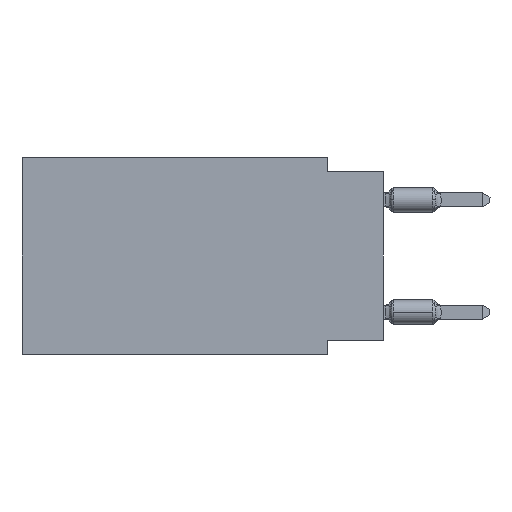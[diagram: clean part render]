
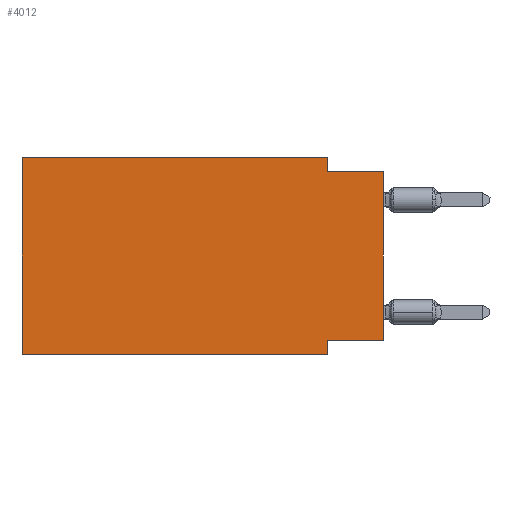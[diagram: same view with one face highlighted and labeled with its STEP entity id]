
A CAD part, left-side view. The second image highlights one B-rep face of the part: STEP entity #4012.
In plain terms, the highlighted planar face has unit normal (-1, 0, 0).
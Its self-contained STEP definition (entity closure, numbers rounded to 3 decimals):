
#630 = VERTEX_POINT ( 'NONE', #11564 ) ;
#721 = CARTESIAN_POINT ( 'NONE',  ( 0., 0., 0. ) ) ;
#818 = ORIENTED_EDGE ( 'NONE', *, *, #9635, .F. ) ;
#1525 = EDGE_CURVE ( 'NONE', #3628, #630, #20084, .T. ) ;
#1866 = EDGE_CURVE ( 'NONE', #13957, #18726, #4700, .T. ) ;
#2178 = EDGE_CURVE ( 'NONE', #13686, #16543, #19381, .T. ) ;
#2636 = VERTEX_POINT ( 'NONE', #3783 ) ;
#2865 = CARTESIAN_POINT ( 'NONE',  ( 0., 0., -8.255 ) ) ;
#2909 = DIRECTION ( 'NONE',  ( 1., 0., 0. ) ) ;
#3628 = VERTEX_POINT ( 'NONE', #11197 ) ;
#3767 = CARTESIAN_POINT ( 'NONE',  ( 0., 0., -0.635 ) ) ;
#3783 = CARTESIAN_POINT ( 'NONE',  ( 0., 2.54, 0. ) ) ;
#4012 = ADVANCED_FACE ( 'NONE', ( #11063 ), #17591, .F. ) ;
#4035 = VECTOR ( 'NONE', #10597, 1000. ) ;
#4369 = EDGE_CURVE ( 'NONE', #2636, #3628, #6198, .T. ) ;
#4674 = CARTESIAN_POINT ( 'NONE',  ( 0., 2.54, -8.89 ) ) ;
#4700 = LINE ( 'NONE', #11255, #20551 ) ;
#5410 = VECTOR ( 'NONE', #14051, 1000. ) ;
#5813 = CARTESIAN_POINT ( 'NONE',  ( 0., 16.383, 0. ) ) ;
#5863 = LINE ( 'NONE', #8883, #18308 ) ;
#5878 = ORIENTED_EDGE ( 'NONE', *, *, #2178, .F. ) ;
#6198 = LINE ( 'NONE', #20715, #5410 ) ;
#7026 = ORIENTED_EDGE ( 'NONE', *, *, #1525, .F. ) ;
#7335 = LINE ( 'NONE', #721, #4035 ) ;
#7657 = VERTEX_POINT ( 'NONE', #13077 ) ;
#7890 = EDGE_LOOP ( 'NONE', ( #16308, #7026, #16889, #818, #18075, #8141, #5878, #11304 ) ) ;
#8141 = ORIENTED_EDGE ( 'NONE', *, *, #18098, .T. ) ;
#8883 = CARTESIAN_POINT ( 'NONE',  ( 0., 16.383, 0. ) ) ;
#9403 = DIRECTION ( 'NONE',  ( 0., 1., 0. ) ) ;
#9521 = LINE ( 'NONE', #2865, #18653 ) ;
#9635 = EDGE_CURVE ( 'NONE', #18726, #2636, #5863, .T. ) ;
#9847 = EDGE_CURVE ( 'NONE', #7657, #13686, #9521, .T. ) ;
#10507 = LINE ( 'NONE', #20803, #12729 ) ;
#10597 = DIRECTION ( 'NONE',  ( 0., 0., 1. ) ) ;
#10920 = DIRECTION ( 'NONE',  ( 0., -1., 0. ) ) ;
#11063 = FACE_OUTER_BOUND ( 'NONE', #7890, .T. ) ;
#11197 = CARTESIAN_POINT ( 'NONE',  ( 0., 2.54, -0.635 ) ) ;
#11255 = CARTESIAN_POINT ( 'NONE',  ( 0., 16.383, 0. ) ) ;
#11304 = ORIENTED_EDGE ( 'NONE', *, *, #9847, .F. ) ;
#11564 = CARTESIAN_POINT ( 'NONE',  ( 0., 0., -0.635 ) ) ;
#12600 = AXIS2_PLACEMENT_3D ( 'NONE', #5813, #2909, #12767 ) ;
#12729 = VECTOR ( 'NONE', #17037, 1000. ) ;
#12746 = CARTESIAN_POINT ( 'NONE',  ( 0., 16.383, -8.89 ) ) ;
#12767 = DIRECTION ( 'NONE',  ( 0., 0., -1. ) ) ;
#13077 = CARTESIAN_POINT ( 'NONE',  ( 0., 0., -8.255 ) ) ;
#13686 = VERTEX_POINT ( 'NONE', #19544 ) ;
#13957 = VERTEX_POINT ( 'NONE', #12746 ) ;
#14051 = DIRECTION ( 'NONE',  ( 0., 0., -1. ) ) ;
#14561 = EDGE_CURVE ( 'NONE', #7657, #630, #7335, .T. ) ;
#16172 = DIRECTION ( 'NONE',  ( 0., 0., 1. ) ) ;
#16308 = ORIENTED_EDGE ( 'NONE', *, *, #14561, .T. ) ;
#16358 = DIRECTION ( 'NONE',  ( 0., 0., -1. ) ) ;
#16543 = VERTEX_POINT ( 'NONE', #19981 ) ;
#16843 = DIRECTION ( 'NONE',  ( 0., -1., 0. ) ) ;
#16889 = ORIENTED_EDGE ( 'NONE', *, *, #4369, .F. ) ;
#17037 = DIRECTION ( 'NONE',  ( 0., -1., 0. ) ) ;
#17591 = PLANE ( 'NONE',  #12600 ) ;
#18075 = ORIENTED_EDGE ( 'NONE', *, *, #1866, .F. ) ;
#18098 = EDGE_CURVE ( 'NONE', #13957, #16543, #10507, .T. ) ;
#18308 = VECTOR ( 'NONE', #10920, 1000. ) ;
#18653 = VECTOR ( 'NONE', #9403, 1000. ) ;
#18726 = VERTEX_POINT ( 'NONE', #19447 ) ;
#19381 = LINE ( 'NONE', #4674, #19393 ) ;
#19393 = VECTOR ( 'NONE', #16358, 1000. ) ;
#19447 = CARTESIAN_POINT ( 'NONE',  ( 0., 16.383, 0. ) ) ;
#19544 = CARTESIAN_POINT ( 'NONE',  ( 0., 2.54, -8.255 ) ) ;
#19981 = CARTESIAN_POINT ( 'NONE',  ( 0., 2.54, -8.89 ) ) ;
#20084 = LINE ( 'NONE', #3767, #20192 ) ;
#20192 = VECTOR ( 'NONE', #16843, 1000. ) ;
#20551 = VECTOR ( 'NONE', #16172, 1000. ) ;
#20715 = CARTESIAN_POINT ( 'NONE',  ( 0., 2.54, 0. ) ) ;
#20803 = CARTESIAN_POINT ( 'NONE',  ( 0., 16.383, -8.89 ) ) ;
